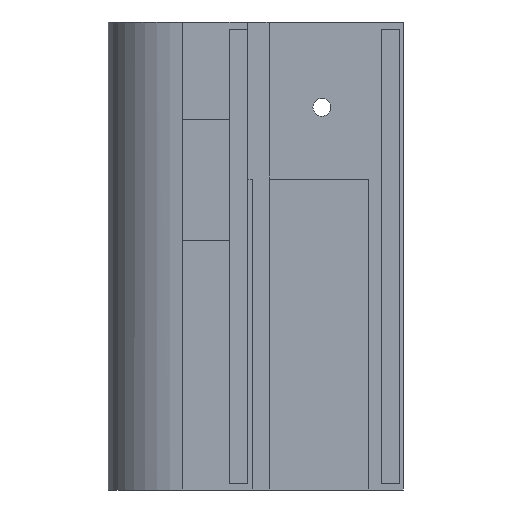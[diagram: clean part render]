
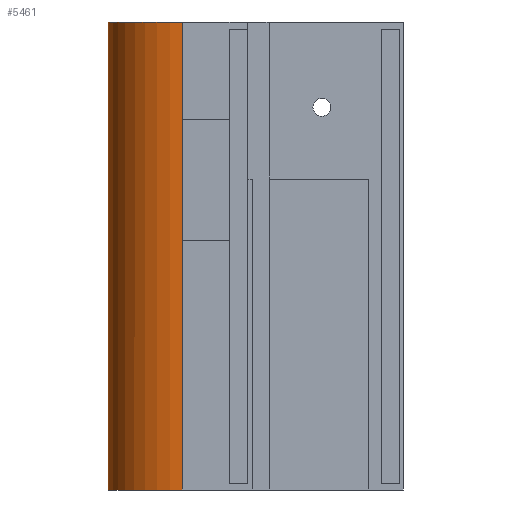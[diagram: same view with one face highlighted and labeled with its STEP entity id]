
A CAD part, left-side view. The second image highlights one B-rep face of the part: STEP entity #5461.
In plain terms, the highlighted cylindrical face has radius 13 mm (diameter 26 mm), a partial arc.
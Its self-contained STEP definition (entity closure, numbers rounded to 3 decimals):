
#1217 = PLANE('',#1218);
#1218 = AXIS2_PLACEMENT_3D('',#1219,#1220,#1221);
#1219 = CARTESIAN_POINT('',(-13.398,41.611,76.189));
#1220 = DIRECTION('',(0.,0.,1.));
#1221 = DIRECTION('',(1.,0.,0.));
#2782 = VERTEX_POINT('',#2783);
#2783 = CARTESIAN_POINT('',(-12.982,25.692,76.189));
#2798 = PLANE('',#2799);
#2799 = AXIS2_PLACEMENT_3D('',#2800,#2801,#2802);
#2800 = CARTESIAN_POINT('',(-18.356,47.561,-1.));
#2801 = DIRECTION('',(0.971,0.239,0.));
#2802 = DIRECTION('',(0.239,-0.971,0.));
#3210 = VERTEX_POINT('',#3211);
#3211 = CARTESIAN_POINT('',(12.986,25.605,76.189));
#3224 = PLANE('',#3225);
#3225 = AXIS2_PLACEMENT_3D('',#3226,#3227,#3228);
#3226 = CARTESIAN_POINT('',(12.986,25.605,-1.));
#3227 = DIRECTION('',(-0.989,0.145,0.));
#3228 = DIRECTION('',(0.145,0.989,0.));
#3235 = EDGE_CURVE('',#2782,#3210,#3236,.T.);
#3236 = SURFACE_CURVE('',#3237,(#3242,#3253),.PCURVE_S1.);
#3237 = CIRCLE('',#3238,13.);
#3238 = AXIS2_PLACEMENT_3D('',#3239,#3240,#3241);
#3239 = CARTESIAN_POINT('',(0.,25.,76.189));
#3240 = DIRECTION('',(0.,0.,-1.));
#3241 = DIRECTION('',(1.,0.,0.));
#3242 = PCURVE('',#1217,#3243);
#3243 = DEFINITIONAL_REPRESENTATION('',(#3244),#3252);
#3244 = ( BOUNDED_CURVE() B_SPLINE_CURVE(2,(#3245,#3246,#3247,#3248,
#3249,#3250,#3251),.UNSPECIFIED.,.T.,.F.) B_SPLINE_CURVE_WITH_KNOTS((1,2
    ,2,2,2,1),(-2.094,0.,2.094,4.189,
6.283,8.378),.UNSPECIFIED.) CURVE() 
GEOMETRIC_REPRESENTATION_ITEM() RATIONAL_B_SPLINE_CURVE((1.,0.5,1.,0.5,
1.,0.5,1.)) REPRESENTATION_ITEM('') );
#3245 = CARTESIAN_POINT('',(26.398,-16.611));
#3246 = CARTESIAN_POINT('',(26.398,-39.127));
#3247 = CARTESIAN_POINT('',(6.898,-27.869));
#3248 = CARTESIAN_POINT('',(-12.602,-16.611));
#3249 = CARTESIAN_POINT('',(6.898,-5.352));
#3250 = CARTESIAN_POINT('',(26.398,5.906));
#3251 = CARTESIAN_POINT('',(26.398,-16.611));
#3252 = ( GEOMETRIC_REPRESENTATION_CONTEXT(2) 
PARAMETRIC_REPRESENTATION_CONTEXT() REPRESENTATION_CONTEXT('2D SPACE',''
  ) );
#3253 = PCURVE('',#3254,#3259);
#3254 = CYLINDRICAL_SURFACE('',#3255,13.);
#3255 = AXIS2_PLACEMENT_3D('',#3256,#3257,#3258);
#3256 = CARTESIAN_POINT('',(0.,25.,-1.));
#3257 = DIRECTION('',(0.,0.,-1.));
#3258 = DIRECTION('',(1.,0.,0.));
#3259 = DEFINITIONAL_REPRESENTATION('',(#3260),#3264);
#3260 = LINE('',#3261,#3262);
#3261 = CARTESIAN_POINT('',(0.,-77.189));
#3262 = VECTOR('',#3263,1.);
#3263 = DIRECTION('',(1.,0.));
#3264 = ( GEOMETRIC_REPRESENTATION_CONTEXT(2) 
PARAMETRIC_REPRESENTATION_CONTEXT() REPRESENTATION_CONTEXT('2D SPACE',''
  ) );
#5342 = VERTEX_POINT('',#5343);
#5343 = CARTESIAN_POINT('',(-12.982,25.692,-1.));
#5357 = PLANE('',#5358);
#5358 = AXIS2_PLACEMENT_3D('',#5359,#5360,#5361);
#5359 = CARTESIAN_POINT('',(-13.,-5.,-1.));
#5360 = DIRECTION('',(0.,0.,-1.));
#5361 = DIRECTION('',(-1.,0.,0.));
#5441 = EDGE_CURVE('',#5342,#2782,#5442,.T.);
#5442 = SURFACE_CURVE('',#5443,(#5447,#5454),.PCURVE_S1.);
#5443 = LINE('',#5444,#5445);
#5444 = CARTESIAN_POINT('',(-12.982,25.692,-1.));
#5445 = VECTOR('',#5446,1.);
#5446 = DIRECTION('',(0.,0.,1.));
#5447 = PCURVE('',#2798,#5448);
#5448 = DEFINITIONAL_REPRESENTATION('',(#5449),#5453);
#5449 = LINE('',#5450,#5451);
#5450 = CARTESIAN_POINT('',(22.52,0.));
#5451 = VECTOR('',#5452,1.);
#5452 = DIRECTION('',(0.,-1.));
#5453 = ( GEOMETRIC_REPRESENTATION_CONTEXT(2) 
PARAMETRIC_REPRESENTATION_CONTEXT() REPRESENTATION_CONTEXT('2D SPACE',''
  ) );
#5454 = PCURVE('',#3254,#5455);
#5455 = DEFINITIONAL_REPRESENTATION('',(#5456),#5460);
#5456 = LINE('',#5457,#5458);
#5457 = CARTESIAN_POINT('',(3.195,0.));
#5458 = VECTOR('',#5459,1.);
#5459 = DIRECTION('',(0.,-1.));
#5460 = ( GEOMETRIC_REPRESENTATION_CONTEXT(2) 
PARAMETRIC_REPRESENTATION_CONTEXT() REPRESENTATION_CONTEXT('2D SPACE',''
  ) );
#5461 = ADVANCED_FACE('',(#5462),#3254,.T.);
#5462 = FACE_BOUND('',#5463,.T.);
#5463 = EDGE_LOOP('',(#5464,#5488,#5489,#5490,#5513,#5542));
#5464 = ORIENTED_EDGE('',*,*,#5465,.F.);
#5465 = EDGE_CURVE('',#5342,#5466,#5468,.T.);
#5466 = VERTEX_POINT('',#5467);
#5467 = CARTESIAN_POINT('',(-11.,31.928,-1.));
#5468 = SURFACE_CURVE('',#5469,(#5474,#5481),.PCURVE_S1.);
#5469 = CIRCLE('',#5470,13.);
#5470 = AXIS2_PLACEMENT_3D('',#5471,#5472,#5473);
#5471 = CARTESIAN_POINT('',(0.,25.,-1.));
#5472 = DIRECTION('',(0.,0.,-1.));
#5473 = DIRECTION('',(1.,0.,0.));
#5474 = PCURVE('',#3254,#5475);
#5475 = DEFINITIONAL_REPRESENTATION('',(#5476),#5480);
#5476 = LINE('',#5477,#5478);
#5477 = CARTESIAN_POINT('',(0.,0.));
#5478 = VECTOR('',#5479,1.);
#5479 = DIRECTION('',(1.,0.));
#5480 = ( GEOMETRIC_REPRESENTATION_CONTEXT(2) 
PARAMETRIC_REPRESENTATION_CONTEXT() REPRESENTATION_CONTEXT('2D SPACE',''
  ) );
#5481 = PCURVE('',#5357,#5482);
#5482 = DEFINITIONAL_REPRESENTATION('',(#5483),#5487);
#5483 = CIRCLE('',#5484,13.);
#5484 = AXIS2_PLACEMENT_2D('',#5485,#5486);
#5485 = CARTESIAN_POINT('',(-13.,30.));
#5486 = DIRECTION('',(-1.,0.));
#5487 = ( GEOMETRIC_REPRESENTATION_CONTEXT(2) 
PARAMETRIC_REPRESENTATION_CONTEXT() REPRESENTATION_CONTEXT('2D SPACE',''
  ) );
#5488 = ORIENTED_EDGE('',*,*,#5441,.T.);
#5489 = ORIENTED_EDGE('',*,*,#3235,.T.);
#5490 = ORIENTED_EDGE('',*,*,#5491,.F.);
#5491 = EDGE_CURVE('',#5492,#3210,#5494,.T.);
#5492 = VERTEX_POINT('',#5493);
#5493 = CARTESIAN_POINT('',(12.986,25.605,-1.));
#5494 = SURFACE_CURVE('',#5495,(#5499,#5506),.PCURVE_S1.);
#5495 = LINE('',#5496,#5497);
#5496 = CARTESIAN_POINT('',(12.986,25.605,-1.));
#5497 = VECTOR('',#5498,1.);
#5498 = DIRECTION('',(0.,0.,1.));
#5499 = PCURVE('',#3254,#5500);
#5500 = DEFINITIONAL_REPRESENTATION('',(#5501),#5505);
#5501 = LINE('',#5502,#5503);
#5502 = CARTESIAN_POINT('',(6.237,0.));
#5503 = VECTOR('',#5504,1.);
#5504 = DIRECTION('',(0.,-1.));
#5505 = ( GEOMETRIC_REPRESENTATION_CONTEXT(2) 
PARAMETRIC_REPRESENTATION_CONTEXT() REPRESENTATION_CONTEXT('2D SPACE',''
  ) );
#5506 = PCURVE('',#3224,#5507);
#5507 = DEFINITIONAL_REPRESENTATION('',(#5508),#5512);
#5508 = LINE('',#5509,#5510);
#5509 = CARTESIAN_POINT('',(0.,0.));
#5510 = VECTOR('',#5511,1.);
#5511 = DIRECTION('',(0.,-1.));
#5512 = ( GEOMETRIC_REPRESENTATION_CONTEXT(2) 
PARAMETRIC_REPRESENTATION_CONTEXT() REPRESENTATION_CONTEXT('2D SPACE',''
  ) );
#5513 = ORIENTED_EDGE('',*,*,#5514,.F.);
#5514 = EDGE_CURVE('',#5515,#5492,#5517,.T.);
#5515 = VERTEX_POINT('',#5516);
#5516 = CARTESIAN_POINT('',(11.,31.928,-1.));
#5517 = SURFACE_CURVE('',#5518,(#5523,#5530),.PCURVE_S1.);
#5518 = CIRCLE('',#5519,13.);
#5519 = AXIS2_PLACEMENT_3D('',#5520,#5521,#5522);
#5520 = CARTESIAN_POINT('',(0.,25.,-1.));
#5521 = DIRECTION('',(0.,0.,-1.));
#5522 = DIRECTION('',(1.,0.,0.));
#5523 = PCURVE('',#3254,#5524);
#5524 = DEFINITIONAL_REPRESENTATION('',(#5525),#5529);
#5525 = LINE('',#5526,#5527);
#5526 = CARTESIAN_POINT('',(0.,0.));
#5527 = VECTOR('',#5528,1.);
#5528 = DIRECTION('',(1.,0.));
#5529 = ( GEOMETRIC_REPRESENTATION_CONTEXT(2) 
PARAMETRIC_REPRESENTATION_CONTEXT() REPRESENTATION_CONTEXT('2D SPACE',''
  ) );
#5530 = PCURVE('',#5531,#5536);
#5531 = PLANE('',#5532);
#5532 = AXIS2_PLACEMENT_3D('',#5533,#5534,#5535);
#5533 = CARTESIAN_POINT('',(-13.,-5.,-1.));
#5534 = DIRECTION('',(0.,0.,-1.));
#5535 = DIRECTION('',(-1.,0.,0.));
#5536 = DEFINITIONAL_REPRESENTATION('',(#5537),#5541);
#5537 = CIRCLE('',#5538,13.);
#5538 = AXIS2_PLACEMENT_2D('',#5539,#5540);
#5539 = CARTESIAN_POINT('',(-13.,30.));
#5540 = DIRECTION('',(-1.,0.));
#5541 = ( GEOMETRIC_REPRESENTATION_CONTEXT(2) 
PARAMETRIC_REPRESENTATION_CONTEXT() REPRESENTATION_CONTEXT('2D SPACE',''
  ) );
#5542 = ORIENTED_EDGE('',*,*,#5543,.F.);
#5543 = EDGE_CURVE('',#5466,#5515,#5544,.T.);
#5544 = SURFACE_CURVE('',#5545,(#5550,#5557),.PCURVE_S1.);
#5545 = CIRCLE('',#5546,13.);
#5546 = AXIS2_PLACEMENT_3D('',#5547,#5548,#5549);
#5547 = CARTESIAN_POINT('',(0.,25.,-1.));
#5548 = DIRECTION('',(0.,0.,-1.));
#5549 = DIRECTION('',(1.,0.,0.));
#5550 = PCURVE('',#3254,#5551);
#5551 = DEFINITIONAL_REPRESENTATION('',(#5552),#5556);
#5552 = LINE('',#5553,#5554);
#5553 = CARTESIAN_POINT('',(0.,0.));
#5554 = VECTOR('',#5555,1.);
#5555 = DIRECTION('',(1.,0.));
#5556 = ( GEOMETRIC_REPRESENTATION_CONTEXT(2) 
PARAMETRIC_REPRESENTATION_CONTEXT() REPRESENTATION_CONTEXT('2D SPACE',''
  ) );
#5557 = PCURVE('',#5558,#5563);
#5558 = PLANE('',#5559);
#5559 = AXIS2_PLACEMENT_3D('',#5560,#5561,#5562);
#5560 = CARTESIAN_POINT('',(-13.,-5.,-1.));
#5561 = DIRECTION('',(0.,0.,-1.));
#5562 = DIRECTION('',(-1.,0.,0.));
#5563 = DEFINITIONAL_REPRESENTATION('',(#5564),#5568);
#5564 = CIRCLE('',#5565,13.);
#5565 = AXIS2_PLACEMENT_2D('',#5566,#5567);
#5566 = CARTESIAN_POINT('',(-13.,30.));
#5567 = DIRECTION('',(-1.,0.));
#5568 = ( GEOMETRIC_REPRESENTATION_CONTEXT(2) 
PARAMETRIC_REPRESENTATION_CONTEXT() REPRESENTATION_CONTEXT('2D SPACE',''
  ) );
